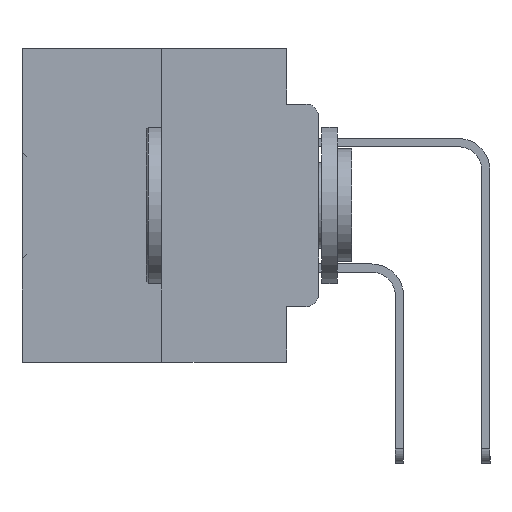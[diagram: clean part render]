
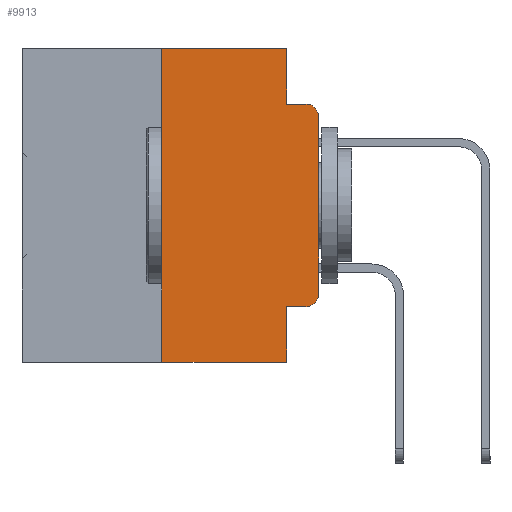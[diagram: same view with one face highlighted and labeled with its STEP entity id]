
A CAD part, left-side view. The second image highlights one B-rep face of the part: STEP entity #9913.
In plain terms, the highlighted planar face has unit normal (-1, 0, 0).
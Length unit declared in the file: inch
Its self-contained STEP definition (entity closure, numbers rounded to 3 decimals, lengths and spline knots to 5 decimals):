
#203 = LINE ( 'NONE', #13702, #14403 ) ;
#291 = EDGE_CURVE ( 'NONE', #27845, #15766, #20606, .T. ) ;
#631 = EDGE_CURVE ( 'NONE', #16029, #35374, #24864, .T. ) ;
#1390 = EDGE_CURVE ( 'NONE', #7153, #19940, #23492, .T. ) ;
#1843 = DIRECTION ( 'NONE',  ( 0., 0., -1. ) ) ;
#2524 = VECTOR ( 'NONE', #1843, 39.37008 ) ;
#3036 = ORIENTED_EDGE ( 'NONE', *, *, #18094, .T. ) ;
#3506 = CARTESIAN_POINT ( 'NONE',  ( 0., 0.473, 0. ) ) ;
#4077 = ORIENTED_EDGE ( 'NONE', *, *, #1390, .T. ) ;
#5547 = EDGE_CURVE ( 'NONE', #19940, #30772, #13684, .T. ) ;
#6341 = DIRECTION ( 'NONE',  ( 0., 0., -1. ) ) ;
#6412 = EDGE_CURVE ( 'NONE', #33126, #16029, #30033, .T. ) ;
#6726 = ORIENTED_EDGE ( 'NONE', *, *, #18092, .T. ) ;
#6745 = LINE ( 'NONE', #18260, #19933 ) ;
#6779 = LINE ( 'NONE', #34028, #19962 ) ;
#7153 = VERTEX_POINT ( 'NONE', #25808 ) ;
#8818 = VERTEX_POINT ( 'NONE', #10136 ) ;
#8828 = CARTESIAN_POINT ( 'NONE',  ( 0., 0.25, -0.5 ) ) ;
#9581 = VECTOR ( 'NONE', #23716, 39.37008 ) ;
#9886 = ORIENTED_EDGE ( 'NONE', *, *, #10925, .F. ) ;
#9913 = ADVANCED_FACE ( 'NONE', ( #24422 ), #17539, .F. ) ;
#9943 = CARTESIAN_POINT ( 'NONE',  ( 0., 0., -0.1085 ) ) ;
#10136 = CARTESIAN_POINT ( 'NONE',  ( 0., 0.051, -0.5 ) ) ;
#10799 = AXIS2_PLACEMENT_3D ( 'NONE', #3506, #23078, #6341 ) ;
#10925 = EDGE_CURVE ( 'NONE', #30217, #33126, #203, .T. ) ;
#11536 = CARTESIAN_POINT ( 'NONE',  ( 0., 0.473, 0. ) ) ;
#11568 = AXIS2_PLACEMENT_3D ( 'NONE', #32847, #16359, #35560 ) ;
#11820 = CARTESIAN_POINT ( 'NONE',  ( 0., 0.02, -0.4115 ) ) ;
#12265 = CARTESIAN_POINT ( 'NONE',  ( 0., 0.051, 0. ) ) ;
#12452 = ORIENTED_EDGE ( 'NONE', *, *, #631, .F. ) ;
#12600 = DIRECTION ( 'NONE',  ( 0., -1., 0. ) ) ;
#13684 = CIRCLE ( 'NONE', #11568, 0.02 ) ;
#13702 = CARTESIAN_POINT ( 'NONE',  ( 0., 0.25, 0. ) ) ;
#14245 = ORIENTED_EDGE ( 'NONE', *, *, #17629, .F. ) ;
#14377 = DIRECTION ( 'NONE',  ( 0., -1., 0. ) ) ;
#14403 = VECTOR ( 'NONE', #19317, 39.37008 ) ;
#15114 = ORIENTED_EDGE ( 'NONE', *, *, #5547, .T. ) ;
#15586 = CARTESIAN_POINT ( 'NONE',  ( 0., 0.02, -0.3915 ) ) ;
#15766 = VERTEX_POINT ( 'NONE', #11820 ) ;
#16029 = VERTEX_POINT ( 'NONE', #32231 ) ;
#16200 = CARTESIAN_POINT ( 'NONE',  ( 0., 0.051, 0. ) ) ;
#16359 = DIRECTION ( 'NONE',  ( -1., 0., 0. ) ) ;
#17096 = ORIENTED_EDGE ( 'NONE', *, *, #291, .T. ) ;
#17539 = PLANE ( 'NONE',  #10799 ) ;
#17575 = DIRECTION ( 'NONE',  ( 0., -1., 0. ) ) ;
#17629 = EDGE_CURVE ( 'NONE', #35374, #30772, #6779, .T. ) ;
#18092 = EDGE_CURVE ( 'NONE', #30217, #8818, #6745, .T. ) ;
#18094 = EDGE_CURVE ( 'NONE', #15766, #7153, #22478, .T. ) ;
#18260 = CARTESIAN_POINT ( 'NONE',  ( 0., 0.473, -0.5 ) ) ;
#18377 = DIRECTION ( 'NONE',  ( 0., 0., -1. ) ) ;
#18932 = AXIS2_PLACEMENT_3D ( 'NONE', #15586, #34821, #18377 ) ;
#19317 = DIRECTION ( 'NONE',  ( 0., 0., 1. ) ) ;
#19590 = CARTESIAN_POINT ( 'NONE',  ( 0., 0.02, -0.0885 ) ) ;
#19933 = VECTOR ( 'NONE', #26572, 39.37008 ) ;
#19940 = VERTEX_POINT ( 'NONE', #9943 ) ;
#19962 = VECTOR ( 'NONE', #17575, 39.37008 ) ;
#20606 = LINE ( 'NONE', #27683, #36000 ) ;
#20655 = CARTESIAN_POINT ( 'NONE',  ( 0., 0.051, -0.0885 ) ) ;
#22478 = CIRCLE ( 'NONE', #18932, 0.02 ) ;
#23078 = DIRECTION ( 'NONE',  ( 1., 0., 0. ) ) ;
#23431 = DIRECTION ( 'NONE',  ( 0., 0., -1. ) ) ;
#23492 = LINE ( 'NONE', #23830, #9581 ) ;
#23716 = DIRECTION ( 'NONE',  ( 0., 0., 1. ) ) ;
#23803 = CARTESIAN_POINT ( 'NONE',  ( 0., 0.25, 0. ) ) ;
#23830 = CARTESIAN_POINT ( 'NONE',  ( 0., 0., 0. ) ) ;
#24422 = FACE_OUTER_BOUND ( 'NONE', #32292, .T. ) ;
#24864 = LINE ( 'NONE', #16200, #2524 ) ;
#25808 = CARTESIAN_POINT ( 'NONE',  ( 0., 0., -0.3915 ) ) ;
#26542 = EDGE_CURVE ( 'NONE', #27845, #8818, #32614, .T. ) ;
#26572 = DIRECTION ( 'NONE',  ( 0., -1., 0. ) ) ;
#27683 = CARTESIAN_POINT ( 'NONE',  ( 0., 0.051, -0.4115 ) ) ;
#27845 = VERTEX_POINT ( 'NONE', #31907 ) ;
#28965 = ORIENTED_EDGE ( 'NONE', *, *, #26542, .F. ) ;
#29187 = VECTOR ( 'NONE', #14377, 39.37008 ) ;
#30033 = LINE ( 'NONE', #11536, #29187 ) ;
#30217 = VERTEX_POINT ( 'NONE', #8828 ) ;
#30772 = VERTEX_POINT ( 'NONE', #19590 ) ;
#31773 = VECTOR ( 'NONE', #23431, 39.37008 ) ;
#31907 = CARTESIAN_POINT ( 'NONE',  ( 0., 0.051, -0.4115 ) ) ;
#32231 = CARTESIAN_POINT ( 'NONE',  ( 0., 0.051, 0. ) ) ;
#32292 = EDGE_LOOP ( 'NONE', ( #4077, #15114, #14245, #12452, #35306, #9886, #6726, #28965, #17096, #3036 ) ) ;
#32614 = LINE ( 'NONE', #12265, #31773 ) ;
#32847 = CARTESIAN_POINT ( 'NONE',  ( 0., 0.02, -0.1085 ) ) ;
#33126 = VERTEX_POINT ( 'NONE', #23803 ) ;
#34028 = CARTESIAN_POINT ( 'NONE',  ( 0., 0.051, -0.0885 ) ) ;
#34821 = DIRECTION ( 'NONE',  ( -1., 0., 0. ) ) ;
#35306 = ORIENTED_EDGE ( 'NONE', *, *, #6412, .F. ) ;
#35374 = VERTEX_POINT ( 'NONE', #20655 ) ;
#35560 = DIRECTION ( 'NONE',  ( 0., 0., -1. ) ) ;
#36000 = VECTOR ( 'NONE', #12600, 39.37008 ) ;
